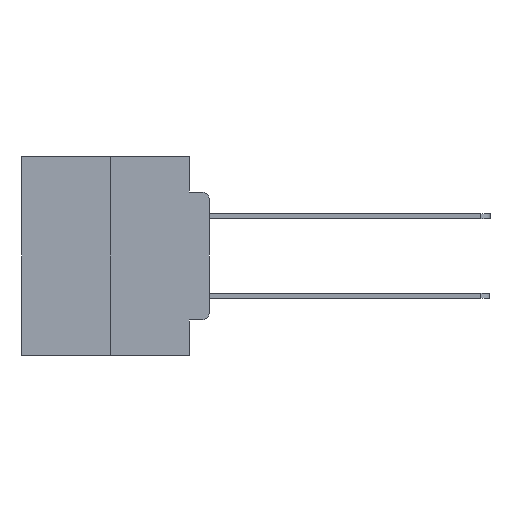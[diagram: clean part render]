
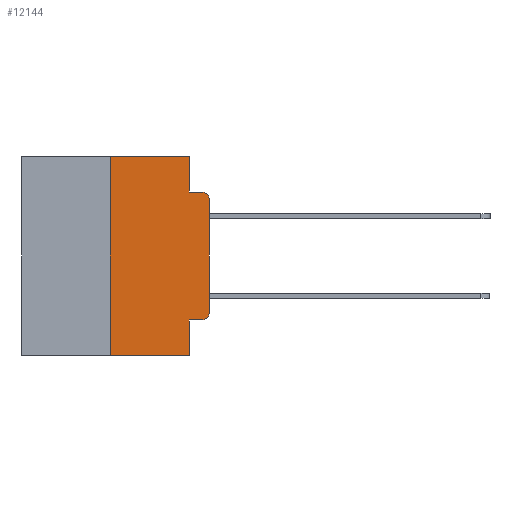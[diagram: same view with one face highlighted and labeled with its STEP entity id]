
A CAD part, left-side view. The second image highlights one B-rep face of the part: STEP entity #12144.
In plain terms, the highlighted planar face has unit normal (-1, 0, 0).
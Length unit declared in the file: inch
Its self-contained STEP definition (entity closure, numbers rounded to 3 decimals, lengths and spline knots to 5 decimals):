
#548 = LINE ( 'NONE', #24147, #16659 ) ;
#926 = EDGE_CURVE ( 'NONE', #24797, #4966, #548, .T. ) ;
#1135 = FACE_OUTER_BOUND ( 'NONE', #4892, .T. ) ;
#1628 = VERTEX_POINT ( 'NONE', #2902 ) ;
#1741 = VECTOR ( 'NONE', #7429, 39.37008 ) ;
#1777 = LINE ( 'NONE', #22832, #23224 ) ;
#1853 = VECTOR ( 'NONE', #26198, 39.37008 ) ;
#2059 = PLANE ( 'NONE',  #7129 ) ;
#2232 = EDGE_CURVE ( 'NONE', #24657, #11590, #23288, .T. ) ;
#2902 = CARTESIAN_POINT ( 'NONE',  ( 0., 0., -0.1085 ) ) ;
#2909 = VECTOR ( 'NONE', #20682, 39.37008 ) ;
#3111 = CARTESIAN_POINT ( 'NONE',  ( 0., 0.051, -0.4115 ) ) ;
#3663 = CARTESIAN_POINT ( 'NONE',  ( 0., 0.051, -0.0885 ) ) ;
#3741 = DIRECTION ( 'NONE',  ( -1., 0., 0. ) ) ;
#3880 = EDGE_CURVE ( 'NONE', #24657, #24203, #6503, .T. ) ;
#4758 = LINE ( 'NONE', #16477, #9676 ) ;
#4781 = CARTESIAN_POINT ( 'NONE',  ( 0., 0.25, 0. ) ) ;
#4892 = EDGE_LOOP ( 'NONE', ( #26577, #24954, #10564, #25925, #15373, #23574, #9900, #12187, #22375, #20508 ) ) ;
#4966 = VERTEX_POINT ( 'NONE', #3663 ) ;
#5185 = CARTESIAN_POINT ( 'NONE',  ( 0., 0.473, 0. ) ) ;
#5959 = CARTESIAN_POINT ( 'NONE',  ( 0., 0.051, 0. ) ) ;
#6183 = DIRECTION ( 'NONE',  ( 0., -1., 0. ) ) ;
#6406 = DIRECTION ( 'NONE',  ( 0., 0., 1. ) ) ;
#6503 = LINE ( 'NONE', #4781, #22233 ) ;
#6555 = VERTEX_POINT ( 'NONE', #12002 ) ;
#6700 = AXIS2_PLACEMENT_3D ( 'NONE', #22572, #11402, #11187 ) ;
#6747 = EDGE_CURVE ( 'NONE', #1628, #6555, #24968, .T. ) ;
#7129 = AXIS2_PLACEMENT_3D ( 'NONE', #14641, #8510, #22839 ) ;
#7429 = DIRECTION ( 'NONE',  ( 0., -1., 0. ) ) ;
#7470 = LINE ( 'NONE', #5185, #1741 ) ;
#8173 = CARTESIAN_POINT ( 'NONE',  ( 0., 0.25, -0.5 ) ) ;
#8510 = DIRECTION ( 'NONE',  ( 1., 0., 0. ) ) ;
#9676 = VECTOR ( 'NONE', #6183, 39.37008 ) ;
#9681 = AXIS2_PLACEMENT_3D ( 'NONE', #16207, #3741, #18243 ) ;
#9748 = LINE ( 'NONE', #5959, #14611 ) ;
#9900 = ORIENTED_EDGE ( 'NONE', *, *, #2232, .T. ) ;
#10564 = ORIENTED_EDGE ( 'NONE', *, *, #10904, .F. ) ;
#10904 = EDGE_CURVE ( 'NONE', #4966, #6555, #20157, .T. ) ;
#11187 = DIRECTION ( 'NONE',  ( 0., 0., -1. ) ) ;
#11402 = DIRECTION ( 'NONE',  ( -1., 0., 0. ) ) ;
#11590 = VERTEX_POINT ( 'NONE', #16626 ) ;
#11805 = CARTESIAN_POINT ( 'NONE',  ( 0., 0.473, -0.5 ) ) ;
#12002 = CARTESIAN_POINT ( 'NONE',  ( 0., 0.02, -0.0885 ) ) ;
#12144 = ADVANCED_FACE ( 'NONE', ( #1135 ), #2059, .F. ) ;
#12187 = ORIENTED_EDGE ( 'NONE', *, *, #25142, .F. ) ;
#13660 = EDGE_CURVE ( 'NONE', #24896, #1628, #1777, .T. ) ;
#14611 = VECTOR ( 'NONE', #26519, 39.37008 ) ;
#14641 = CARTESIAN_POINT ( 'NONE',  ( 0., 0.473, 0. ) ) ;
#15167 = VERTEX_POINT ( 'NONE', #3111 ) ;
#15373 = ORIENTED_EDGE ( 'NONE', *, *, #16523, .F. ) ;
#16207 = CARTESIAN_POINT ( 'NONE',  ( 0., 0.02, -0.3915 ) ) ;
#16477 = CARTESIAN_POINT ( 'NONE',  ( 0., 0.051, -0.4115 ) ) ;
#16523 = EDGE_CURVE ( 'NONE', #24203, #24797, #7470, .T. ) ;
#16626 = CARTESIAN_POINT ( 'NONE',  ( 0., 0.051, -0.5 ) ) ;
#16659 = VECTOR ( 'NONE', #26816, 39.37008 ) ;
#17687 = CIRCLE ( 'NONE', #9681, 0.02 ) ;
#17719 = DIRECTION ( 'NONE',  ( 0., 0., 1. ) ) ;
#17832 = CARTESIAN_POINT ( 'NONE',  ( 0., 0.02, -0.4115 ) ) ;
#18243 = DIRECTION ( 'NONE',  ( 0., 0., -1. ) ) ;
#18990 = CARTESIAN_POINT ( 'NONE',  ( 0., 0.25, 0. ) ) ;
#19598 = CARTESIAN_POINT ( 'NONE',  ( 0., 0., -0.3915 ) ) ;
#20157 = LINE ( 'NONE', #24696, #2909 ) ;
#20508 = ORIENTED_EDGE ( 'NONE', *, *, #21026, .T. ) ;
#20682 = DIRECTION ( 'NONE',  ( 0., -1., 0. ) ) ;
#21026 = EDGE_CURVE ( 'NONE', #22890, #24896, #17687, .T. ) ;
#22233 = VECTOR ( 'NONE', #17719, 39.37008 ) ;
#22375 = ORIENTED_EDGE ( 'NONE', *, *, #26500, .T. ) ;
#22572 = CARTESIAN_POINT ( 'NONE',  ( 0., 0.02, -0.1085 ) ) ;
#22832 = CARTESIAN_POINT ( 'NONE',  ( 0., 0., 0. ) ) ;
#22839 = DIRECTION ( 'NONE',  ( 0., 0., -1. ) ) ;
#22890 = VERTEX_POINT ( 'NONE', #17832 ) ;
#23224 = VECTOR ( 'NONE', #6406, 39.37008 ) ;
#23288 = LINE ( 'NONE', #11805, #1853 ) ;
#23406 = CARTESIAN_POINT ( 'NONE',  ( 0., 0.051, 0. ) ) ;
#23574 = ORIENTED_EDGE ( 'NONE', *, *, #3880, .F. ) ;
#24147 = CARTESIAN_POINT ( 'NONE',  ( 0., 0.051, 0. ) ) ;
#24203 = VERTEX_POINT ( 'NONE', #18990 ) ;
#24657 = VERTEX_POINT ( 'NONE', #8173 ) ;
#24696 = CARTESIAN_POINT ( 'NONE',  ( 0., 0.051, -0.0885 ) ) ;
#24797 = VERTEX_POINT ( 'NONE', #23406 ) ;
#24896 = VERTEX_POINT ( 'NONE', #19598 ) ;
#24954 = ORIENTED_EDGE ( 'NONE', *, *, #6747, .T. ) ;
#24968 = CIRCLE ( 'NONE', #6700, 0.02 ) ;
#25142 = EDGE_CURVE ( 'NONE', #15167, #11590, #9748, .T. ) ;
#25925 = ORIENTED_EDGE ( 'NONE', *, *, #926, .F. ) ;
#26198 = DIRECTION ( 'NONE',  ( 0., -1., 0. ) ) ;
#26500 = EDGE_CURVE ( 'NONE', #15167, #22890, #4758, .T. ) ;
#26519 = DIRECTION ( 'NONE',  ( 0., 0., -1. ) ) ;
#26577 = ORIENTED_EDGE ( 'NONE', *, *, #13660, .T. ) ;
#26816 = DIRECTION ( 'NONE',  ( 0., 0., -1. ) ) ;
